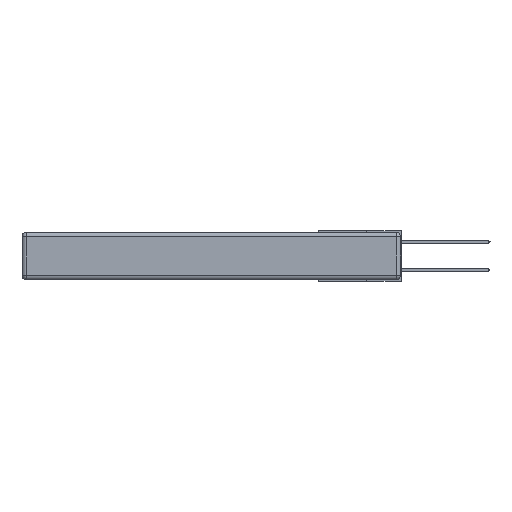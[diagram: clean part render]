
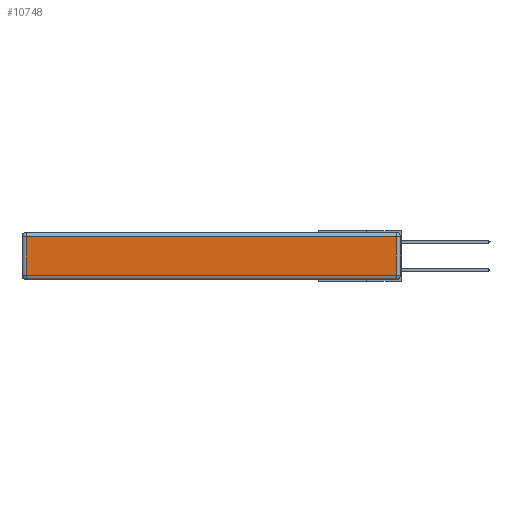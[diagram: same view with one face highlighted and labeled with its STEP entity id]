
A CAD part, left-side view. The second image highlights one B-rep face of the part: STEP entity #10748.
In plain terms, the highlighted planar face has unit normal (-1, 0, 0).
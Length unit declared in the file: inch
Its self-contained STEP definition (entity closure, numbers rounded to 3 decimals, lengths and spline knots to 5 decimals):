
#594 = ORIENTED_EDGE ( 'NONE', *, *, #35082, .T. ) ;
#783 = EDGE_LOOP ( 'NONE', ( #30952, #4483, #24289, #594 ) ) ;
#1178 = DIRECTION ( 'NONE',  ( 0., 0., 1. ) ) ;
#3842 = LINE ( 'NONE', #33714, #32020 ) ;
#4483 = ORIENTED_EDGE ( 'NONE', *, *, #34538, .T. ) ;
#5078 = VECTOR ( 'NONE', #26779, 39.37008 ) ;
#5111 = LINE ( 'NONE', #31779, #11500 ) ;
#7963 = CARTESIAN_POINT ( 'NONE',  ( 0., 0.03, -0.313 ) ) ;
#8460 = EDGE_CURVE ( 'NONE', #14476, #13267, #5111, .T. ) ;
#10111 = CARTESIAN_POINT ( 'NONE',  ( 0., 0.03, -0.03 ) ) ;
#10748 = ADVANCED_FACE ( 'NONE', ( #19393 ), #28322, .T. ) ;
#11500 = VECTOR ( 'NONE', #15380, 39.37008 ) ;
#13267 = VERTEX_POINT ( 'NONE', #15515 ) ;
#14011 = LINE ( 'NONE', #26431, #5078 ) ;
#14476 = VERTEX_POINT ( 'NONE', #10111 ) ;
#15380 = DIRECTION ( 'NONE',  ( 0., 1., 0. ) ) ;
#15515 = CARTESIAN_POINT ( 'NONE',  ( 0., 2.72, -0.03 ) ) ;
#18506 = AXIS2_PLACEMENT_3D ( 'NONE', #23015, #34046, #1178 ) ;
#19393 = FACE_OUTER_BOUND ( 'NONE', #783, .T. ) ;
#19642 = DIRECTION ( 'NONE',  ( 0., 0., -1. ) ) ;
#20805 = VECTOR ( 'NONE', #19642, 39.37008 ) ;
#23015 = CARTESIAN_POINT ( 'NONE',  ( 0., 0., -0.343 ) ) ;
#24289 = ORIENTED_EDGE ( 'NONE', *, *, #8460, .T. ) ;
#24676 = VERTEX_POINT ( 'NONE', #7963 ) ;
#26431 = CARTESIAN_POINT ( 'NONE',  ( 0., 0.03, -0.343 ) ) ;
#26779 = DIRECTION ( 'NONE',  ( 0., 0., 1. ) ) ;
#28135 = LINE ( 'NONE', #30904, #20805 ) ;
#28322 = PLANE ( 'NONE',  #18506 ) ;
#28457 = CARTESIAN_POINT ( 'NONE',  ( 0., 2.72, -0.313 ) ) ;
#30105 = EDGE_CURVE ( 'NONE', #33635, #24676, #3842, .T. ) ;
#30904 = CARTESIAN_POINT ( 'NONE',  ( 0., 2.72, -0.343 ) ) ;
#30952 = ORIENTED_EDGE ( 'NONE', *, *, #30105, .T. ) ;
#31063 = DIRECTION ( 'NONE',  ( 0., -1., 0. ) ) ;
#31779 = CARTESIAN_POINT ( 'NONE',  ( 0., 2.75, -0.03 ) ) ;
#32020 = VECTOR ( 'NONE', #31063, 39.37008 ) ;
#33635 = VERTEX_POINT ( 'NONE', #28457 ) ;
#33714 = CARTESIAN_POINT ( 'NONE',  ( 0., 0., -0.313 ) ) ;
#34046 = DIRECTION ( 'NONE',  ( -1., 0., 0. ) ) ;
#34538 = EDGE_CURVE ( 'NONE', #24676, #14476, #14011, .T. ) ;
#35082 = EDGE_CURVE ( 'NONE', #13267, #33635, #28135, .T. ) ;
